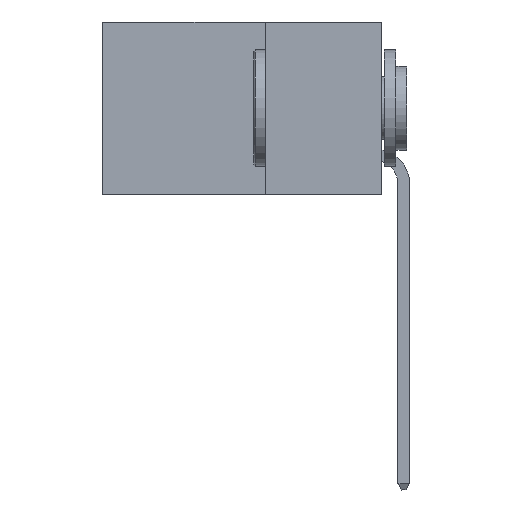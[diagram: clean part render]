
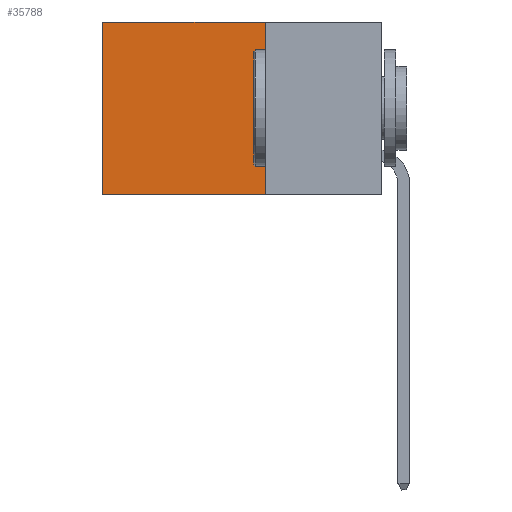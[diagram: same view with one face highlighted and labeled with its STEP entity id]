
A CAD part, left-side view. The second image highlights one B-rep face of the part: STEP entity #35788.
In plain terms, the highlighted planar face has unit normal (-1, 0, 0).
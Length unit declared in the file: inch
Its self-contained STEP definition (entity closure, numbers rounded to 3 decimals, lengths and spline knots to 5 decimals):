
#99 = EDGE_LOOP ( 'NONE', ( #8224, #17945, #26448, #17248 ) ) ;
#377 = VERTEX_POINT ( 'NONE', #6623 ) ;
#734 = CARTESIAN_POINT ( 'NONE',  ( 0.2875, 0.25, 0. ) ) ;
#892 = PLANE ( 'NONE',  #3544 ) ;
#1165 = DIRECTION ( 'NONE',  ( 0., 0., -1. ) ) ;
#1578 = DIRECTION ( 'NONE',  ( 0., 1., 0. ) ) ;
#2123 = EDGE_CURVE ( 'NONE', #377, #7202, #6140, .T. ) ;
#2482 = FACE_OUTER_BOUND ( 'NONE', #99, .T. ) ;
#3544 = AXIS2_PLACEMENT_3D ( 'NONE', #3672, #23160, #6452 ) ;
#3632 = DIRECTION ( 'NONE',  ( 0., 1., 0. ) ) ;
#3672 = CARTESIAN_POINT ( 'NONE',  ( 0.2875, 0.25, 0. ) ) ;
#3802 = LINE ( 'NONE', #734, #32585 ) ;
#4239 = LINE ( 'NONE', #18267, #19104 ) ;
#5274 = VECTOR ( 'NONE', #24885, 39.37008 ) ;
#6140 = LINE ( 'NONE', #33050, #5274 ) ;
#6452 = DIRECTION ( 'NONE',  ( 0., 0., -1. ) ) ;
#6623 = CARTESIAN_POINT ( 'NONE',  ( 0.2875, 0.6, 0. ) ) ;
#7202 = VERTEX_POINT ( 'NONE', #23568 ) ;
#8224 = ORIENTED_EDGE ( 'NONE', *, *, #2123, .T. ) ;
#8711 = EDGE_CURVE ( 'NONE', #33702, #377, #3802, .T. ) ;
#8804 = CARTESIAN_POINT ( 'NONE',  ( 0.2875, 0.25, -0.37 ) ) ;
#10178 = VECTOR ( 'NONE', #1165, 39.37008 ) ;
#15629 = EDGE_CURVE ( 'NONE', #33702, #17972, #32404, .T. ) ;
#17248 = ORIENTED_EDGE ( 'NONE', *, *, #8711, .T. ) ;
#17945 = ORIENTED_EDGE ( 'NONE', *, *, #27575, .F. ) ;
#17972 = VERTEX_POINT ( 'NONE', #8804 ) ;
#18267 = CARTESIAN_POINT ( 'NONE',  ( 0.2875, 0.25, -0.37 ) ) ;
#19104 = VECTOR ( 'NONE', #1578, 39.37008 ) ;
#23160 = DIRECTION ( 'NONE',  ( 1., 0., 0. ) ) ;
#23568 = CARTESIAN_POINT ( 'NONE',  ( 0.2875, 0.6, -0.37 ) ) ;
#24885 = DIRECTION ( 'NONE',  ( 0., 0., -1. ) ) ;
#26095 = CARTESIAN_POINT ( 'NONE',  ( 0.2875, 0.25, 0. ) ) ;
#26448 = ORIENTED_EDGE ( 'NONE', *, *, #15629, .F. ) ;
#27575 = EDGE_CURVE ( 'NONE', #17972, #7202, #4239, .T. ) ;
#32404 = LINE ( 'NONE', #26095, #10178 ) ;
#32585 = VECTOR ( 'NONE', #3632, 39.37008 ) ;
#33050 = CARTESIAN_POINT ( 'NONE',  ( 0.2875, 0.6, 0. ) ) ;
#33320 = CARTESIAN_POINT ( 'NONE',  ( 0.2875, 0.25, 0. ) ) ;
#33702 = VERTEX_POINT ( 'NONE', #33320 ) ;
#35788 = ADVANCED_FACE ( 'NONE', ( #2482 ), #892, .F. ) ;
